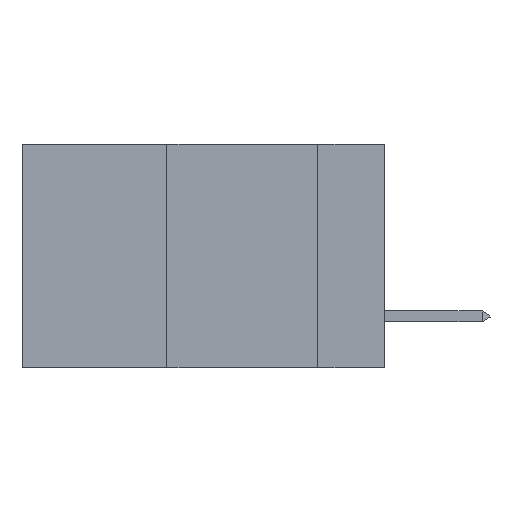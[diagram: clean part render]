
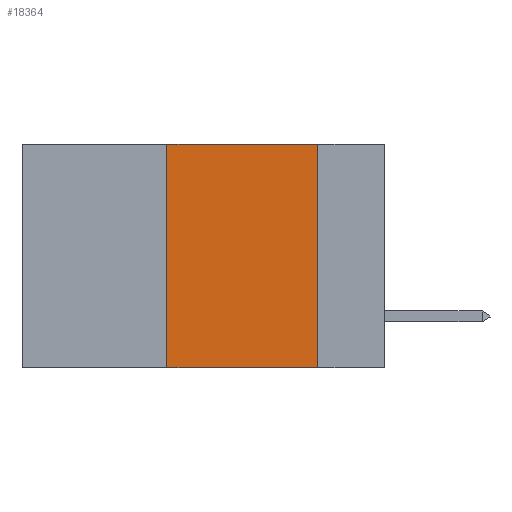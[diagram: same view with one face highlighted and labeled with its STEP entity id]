
A CAD part, left-side view. The second image highlights one B-rep face of the part: STEP entity #18364.
In plain terms, the highlighted planar face has unit normal (-1, 0, 0).
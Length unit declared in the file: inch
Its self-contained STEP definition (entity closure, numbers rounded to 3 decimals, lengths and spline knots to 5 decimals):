
#1704 = LINE ( 'NONE', #20154, #17595 ) ;
#2115 = ORIENTED_EDGE ( 'NONE', *, *, #14997, .F. ) ;
#3084 = DIRECTION ( 'NONE',  ( 0., 0., -1. ) ) ;
#3397 = DIRECTION ( 'NONE',  ( 1., 0., 0. ) ) ;
#3398 = AXIS2_PLACEMENT_3D ( 'NONE', #6899, #3397, #13758 ) ;
#4947 = VERTEX_POINT ( 'NONE', #8336 ) ;
#5682 = ORIENTED_EDGE ( 'NONE', *, *, #8982, .F. ) ;
#6882 = ORIENTED_EDGE ( 'NONE', *, *, #14922, .F. ) ;
#6896 = LINE ( 'NONE', #9396, #21262 ) ;
#6899 = CARTESIAN_POINT ( 'NONE',  ( 0., 0.6, 0. ) ) ;
#8237 = CARTESIAN_POINT ( 'NONE',  ( 0., 0.36, -0.37 ) ) ;
#8336 = CARTESIAN_POINT ( 'NONE',  ( 0., 0.36, 0. ) ) ;
#8982 = EDGE_CURVE ( 'NONE', #4947, #16977, #13113, .T. ) ;
#9396 = CARTESIAN_POINT ( 'NONE',  ( 0., 0.6, -0.37 ) ) ;
#11211 = VECTOR ( 'NONE', #3084, 39.37008 ) ;
#11577 = CARTESIAN_POINT ( 'NONE',  ( 0., 0.11, -0.37 ) ) ;
#11993 = DIRECTION ( 'NONE',  ( 0., 0., 1. ) ) ;
#12929 = ORIENTED_EDGE ( 'NONE', *, *, #16986, .T. ) ;
#13113 = LINE ( 'NONE', #17980, #19005 ) ;
#13254 = PLANE ( 'NONE',  #3398 ) ;
#13327 = VERTEX_POINT ( 'NONE', #8237 ) ;
#13337 = EDGE_LOOP ( 'NONE', ( #2115, #5682, #6882, #12929 ) ) ;
#13758 = DIRECTION ( 'NONE',  ( 0., 0., -1. ) ) ;
#14922 = EDGE_CURVE ( 'NONE', #13327, #4947, #1704, .T. ) ;
#14997 = EDGE_CURVE ( 'NONE', #16977, #20676, #15589, .T. ) ;
#15589 = LINE ( 'NONE', #20073, #11211 ) ;
#16977 = VERTEX_POINT ( 'NONE', #17493 ) ;
#16986 = EDGE_CURVE ( 'NONE', #13327, #20676, #6896, .T. ) ;
#17493 = CARTESIAN_POINT ( 'NONE',  ( 0., 0.11, 0. ) ) ;
#17595 = VECTOR ( 'NONE', #11993, 39.37008 ) ;
#17980 = CARTESIAN_POINT ( 'NONE',  ( 0., 0.6, 0. ) ) ;
#18364 = ADVANCED_FACE ( 'NONE', ( #19944 ), #13254, .F. ) ;
#19005 = VECTOR ( 'NONE', #19473, 39.37008 ) ;
#19336 = DIRECTION ( 'NONE',  ( 0., -1., 0. ) ) ;
#19473 = DIRECTION ( 'NONE',  ( 0., -1., 0. ) ) ;
#19944 = FACE_OUTER_BOUND ( 'NONE', #13337, .T. ) ;
#20073 = CARTESIAN_POINT ( 'NONE',  ( 0., 0.11, 0. ) ) ;
#20154 = CARTESIAN_POINT ( 'NONE',  ( 0., 0.36, 0. ) ) ;
#20676 = VERTEX_POINT ( 'NONE', #11577 ) ;
#21262 = VECTOR ( 'NONE', #19336, 39.37008 ) ;
